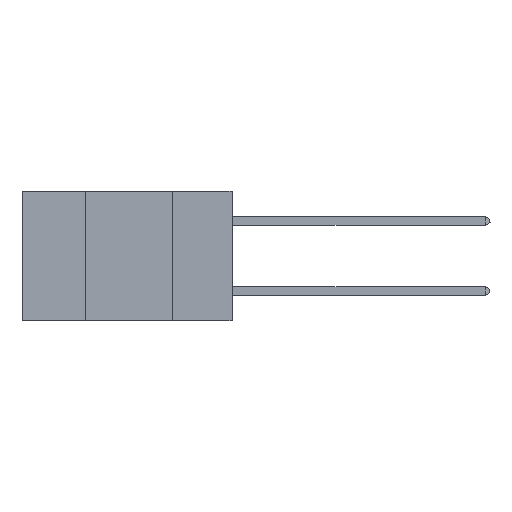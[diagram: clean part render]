
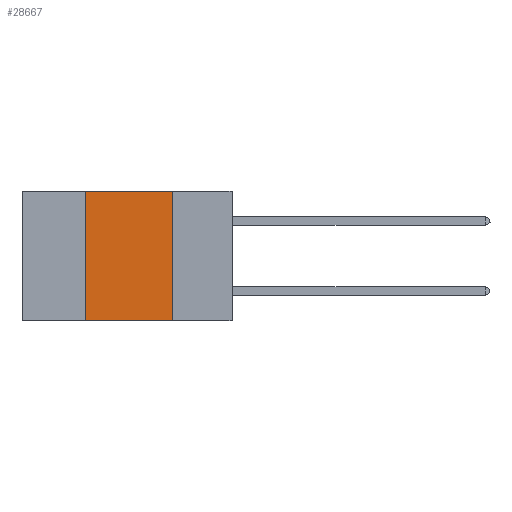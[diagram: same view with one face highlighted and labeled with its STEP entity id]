
A CAD part, left-side view. The second image highlights one B-rep face of the part: STEP entity #28667.
In plain terms, the highlighted planar face has unit normal (-1, 0, 0).
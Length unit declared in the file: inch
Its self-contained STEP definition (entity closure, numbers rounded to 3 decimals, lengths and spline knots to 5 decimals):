
#299 = ORIENTED_EDGE ( 'NONE', *, *, #9731, .F. ) ;
#1847 = DIRECTION ( 'NONE',  ( 0., 0., 1. ) ) ;
#2081 = CARTESIAN_POINT ( 'NONE',  ( 0., 0.17, 0. ) ) ;
#2276 = ORIENTED_EDGE ( 'NONE', *, *, #28569, .F. ) ;
#2608 = DIRECTION ( 'NONE',  ( 0., 0., -1. ) ) ;
#3689 = VERTEX_POINT ( 'NONE', #23519 ) ;
#4409 = CARTESIAN_POINT ( 'NONE',  ( 0., 0.17, 0. ) ) ;
#5357 = ORIENTED_EDGE ( 'NONE', *, *, #10381, .F. ) ;
#6891 = VECTOR ( 'NONE', #18175, 39.37008 ) ;
#7037 = LINE ( 'NONE', #18311, #32656 ) ;
#9731 = EDGE_CURVE ( 'NONE', #3689, #34854, #7037, .T. ) ;
#10381 = EDGE_CURVE ( 'NONE', #34854, #34571, #24329, .T. ) ;
#10854 = FACE_OUTER_BOUND ( 'NONE', #23403, .T. ) ;
#13623 = CARTESIAN_POINT ( 'NONE',  ( 0., 0.6, 0. ) ) ;
#13960 = CARTESIAN_POINT ( 'NONE',  ( 0., 0.17, -0.37 ) ) ;
#16369 = VERTEX_POINT ( 'NONE', #13960 ) ;
#17844 = VECTOR ( 'NONE', #27186, 39.37008 ) ;
#18175 = DIRECTION ( 'NONE',  ( 0., 0., -1. ) ) ;
#18311 = CARTESIAN_POINT ( 'NONE',  ( 0., 0.42, 0. ) ) ;
#18622 = LINE ( 'NONE', #32362, #19961 ) ;
#19961 = VECTOR ( 'NONE', #21485, 39.37008 ) ;
#20422 = EDGE_CURVE ( 'NONE', #3689, #16369, #18622, .T. ) ;
#21485 = DIRECTION ( 'NONE',  ( 0., -1., 0. ) ) ;
#21923 = DIRECTION ( 'NONE',  ( 1., 0., 0. ) ) ;
#22315 = AXIS2_PLACEMENT_3D ( 'NONE', #27091, #21923, #2608 ) ;
#23329 = CARTESIAN_POINT ( 'NONE',  ( 0., 0.42, 0. ) ) ;
#23403 = EDGE_LOOP ( 'NONE', ( #2276, #5357, #299, #32239 ) ) ;
#23519 = CARTESIAN_POINT ( 'NONE',  ( 0., 0.42, -0.37 ) ) ;
#23888 = LINE ( 'NONE', #4409, #6891 ) ;
#24329 = LINE ( 'NONE', #13623, #17844 ) ;
#26917 = PLANE ( 'NONE',  #22315 ) ;
#27091 = CARTESIAN_POINT ( 'NONE',  ( 0., 0.6, 0. ) ) ;
#27186 = DIRECTION ( 'NONE',  ( 0., -1., 0. ) ) ;
#28569 = EDGE_CURVE ( 'NONE', #34571, #16369, #23888, .T. ) ;
#28667 = ADVANCED_FACE ( 'NONE', ( #10854 ), #26917, .F. ) ;
#32239 = ORIENTED_EDGE ( 'NONE', *, *, #20422, .T. ) ;
#32362 = CARTESIAN_POINT ( 'NONE',  ( 0., 0.6, -0.37 ) ) ;
#32656 = VECTOR ( 'NONE', #1847, 39.37008 ) ;
#34571 = VERTEX_POINT ( 'NONE', #2081 ) ;
#34854 = VERTEX_POINT ( 'NONE', #23329 ) ;
